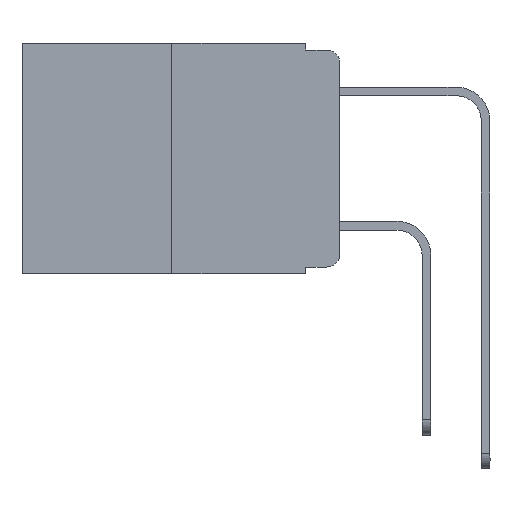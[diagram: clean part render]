
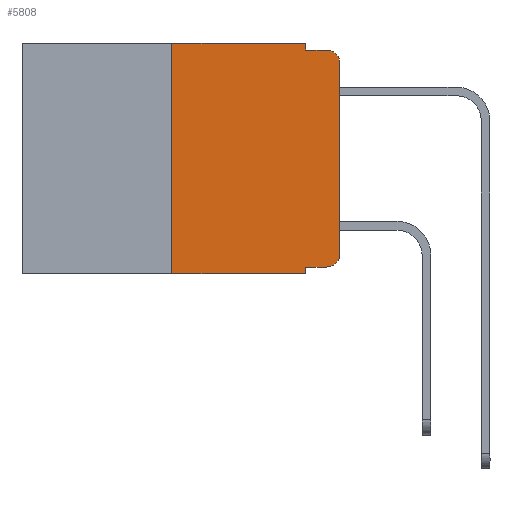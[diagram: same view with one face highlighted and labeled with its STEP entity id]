
A CAD part, left-side view. The second image highlights one B-rep face of the part: STEP entity #5808.
In plain terms, the highlighted planar face has unit normal (-1, 0, 0).
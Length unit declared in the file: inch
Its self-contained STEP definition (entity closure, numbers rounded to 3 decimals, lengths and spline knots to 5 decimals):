
#131 = CARTESIAN_POINT ( 'NONE',  ( 0., 0.02, -0.333 ) ) ;
#281 = CARTESIAN_POINT ( 'NONE',  ( 0., 0.473, 0. ) ) ;
#1119 = DIRECTION ( 'NONE',  ( 0., -1., 0. ) ) ;
#1161 = LINE ( 'NONE', #17422, #10593 ) ;
#2213 = EDGE_CURVE ( 'NONE', #14482, #23473, #11950, .T. ) ;
#2402 = EDGE_CURVE ( 'NONE', #11995, #22808, #20182, .T. ) ;
#2594 = VECTOR ( 'NONE', #10227, 39.37008 ) ;
#2926 = DIRECTION ( 'NONE',  ( 0., 0., -1. ) ) ;
#3239 = EDGE_CURVE ( 'NONE', #14482, #4214, #15384, .T. ) ;
#3507 = VECTOR ( 'NONE', #1119, 39.37008 ) ;
#3679 = CARTESIAN_POINT ( 'NONE',  ( 0., 0.051, -0.333 ) ) ;
#3742 = CIRCLE ( 'NONE', #18759, 0.02 ) ;
#4099 = VERTEX_POINT ( 'NONE', #24246 ) ;
#4214 = VERTEX_POINT ( 'NONE', #25661 ) ;
#5206 = DIRECTION ( 'NONE',  ( 0., 0., -1. ) ) ;
#5703 = LINE ( 'NONE', #21969, #22738 ) ;
#5708 = ORIENTED_EDGE ( 'NONE', *, *, #2402, .T. ) ;
#5808 = ADVANCED_FACE ( 'NONE', ( #22714 ), #18697, .F. ) ;
#6368 = ORIENTED_EDGE ( 'NONE', *, *, #11559, .F. ) ;
#6681 = VECTOR ( 'NONE', #22497, 39.37008 ) ;
#6683 = EDGE_CURVE ( 'NONE', #16133, #4099, #24520, .T. ) ;
#7158 = CARTESIAN_POINT ( 'NONE',  ( 0., 0.051, -0.01 ) ) ;
#7384 = ORIENTED_EDGE ( 'NONE', *, *, #6683, .F. ) ;
#7598 = DIRECTION ( 'NONE',  ( 0., 0., -1. ) ) ;
#8269 = VECTOR ( 'NONE', #2926, 39.37008 ) ;
#8389 = VERTEX_POINT ( 'NONE', #9646 ) ;
#8846 = ORIENTED_EDGE ( 'NONE', *, *, #21223, .F. ) ;
#9257 = CARTESIAN_POINT ( 'NONE',  ( 0., 0.02, -0.03 ) ) ;
#9646 = CARTESIAN_POINT ( 'NONE',  ( 0., 0., -0.313 ) ) ;
#9952 = CARTESIAN_POINT ( 'NONE',  ( 0., 0.051, -0.333 ) ) ;
#10069 = EDGE_LOOP ( 'NONE', ( #24864, #5708, #21512, #6368, #7384, #8846, #12903, #10584, #22811, #16232 ) ) ;
#10111 = DIRECTION ( 'NONE',  ( 0., 0., -1. ) ) ;
#10227 = DIRECTION ( 'NONE',  ( 0., -1., 0. ) ) ;
#10337 = EDGE_CURVE ( 'NONE', #22990, #22808, #19526, .T. ) ;
#10584 = ORIENTED_EDGE ( 'NONE', *, *, #3239, .F. ) ;
#10593 = VECTOR ( 'NONE', #23998, 39.37008 ) ;
#11559 = EDGE_CURVE ( 'NONE', #4099, #22990, #5703, .T. ) ;
#11950 = LINE ( 'NONE', #9952, #2594 ) ;
#11995 = VERTEX_POINT ( 'NONE', #26079 ) ;
#12903 = ORIENTED_EDGE ( 'NONE', *, *, #26313, .T. ) ;
#13415 = DIRECTION ( 'NONE',  ( 0., 0., 1. ) ) ;
#13844 = VECTOR ( 'NONE', #13415, 39.37008 ) ;
#14438 = LINE ( 'NONE', #19959, #25424 ) ;
#14482 = VERTEX_POINT ( 'NONE', #3679 ) ;
#15384 = LINE ( 'NONE', #23603, #8269 ) ;
#15413 = LINE ( 'NONE', #23634, #13844 ) ;
#15506 = DIRECTION ( 'NONE',  ( 0., 0., -1. ) ) ;
#15543 = DIRECTION ( 'NONE',  ( -1., 0., 0. ) ) ;
#16031 = AXIS2_PLACEMENT_3D ( 'NONE', #281, #24481, #10111 ) ;
#16133 = VERTEX_POINT ( 'NONE', #19725 ) ;
#16232 = ORIENTED_EDGE ( 'NONE', *, *, #25167, .T. ) ;
#16446 = CARTESIAN_POINT ( 'NONE',  ( 0., 0.473, 0. ) ) ;
#17422 = CARTESIAN_POINT ( 'NONE',  ( 0., 0.473, -0.343 ) ) ;
#17816 = CARTESIAN_POINT ( 'NONE',  ( 0., 0.02, -0.313 ) ) ;
#18697 = PLANE ( 'NONE',  #16031 ) ;
#18759 = AXIS2_PLACEMENT_3D ( 'NONE', #17816, #26019, #7598 ) ;
#19340 = EDGE_CURVE ( 'NONE', #8389, #11995, #15413, .T. ) ;
#19526 = LINE ( 'NONE', #7158, #3507 ) ;
#19725 = CARTESIAN_POINT ( 'NONE',  ( 0., 0.25, 0. ) ) ;
#19959 = CARTESIAN_POINT ( 'NONE',  ( 0., 0.25, 0. ) ) ;
#20088 = DIRECTION ( 'NONE',  ( 0., 0., 1. ) ) ;
#20182 = CIRCLE ( 'NONE', #26208, 0.02 ) ;
#20976 = CARTESIAN_POINT ( 'NONE',  ( 0., 0.051, -0.01 ) ) ;
#21223 = EDGE_CURVE ( 'NONE', #23189, #16133, #14438, .T. ) ;
#21512 = ORIENTED_EDGE ( 'NONE', *, *, #10337, .F. ) ;
#21969 = CARTESIAN_POINT ( 'NONE',  ( 0., 0.051, 0. ) ) ;
#22497 = DIRECTION ( 'NONE',  ( 0., -1., 0. ) ) ;
#22714 = FACE_OUTER_BOUND ( 'NONE', #10069, .T. ) ;
#22738 = VECTOR ( 'NONE', #15506, 39.37008 ) ;
#22808 = VERTEX_POINT ( 'NONE', #25442 ) ;
#22811 = ORIENTED_EDGE ( 'NONE', *, *, #2213, .T. ) ;
#22990 = VERTEX_POINT ( 'NONE', #20976 ) ;
#23189 = VERTEX_POINT ( 'NONE', #23521 ) ;
#23473 = VERTEX_POINT ( 'NONE', #131 ) ;
#23521 = CARTESIAN_POINT ( 'NONE',  ( 0., 0.25, -0.343 ) ) ;
#23603 = CARTESIAN_POINT ( 'NONE',  ( 0., 0.051, 0. ) ) ;
#23634 = CARTESIAN_POINT ( 'NONE',  ( 0., 0., 0. ) ) ;
#23998 = DIRECTION ( 'NONE',  ( 0., -1., 0. ) ) ;
#24246 = CARTESIAN_POINT ( 'NONE',  ( 0., 0.051, 0. ) ) ;
#24481 = DIRECTION ( 'NONE',  ( 1., 0., 0. ) ) ;
#24520 = LINE ( 'NONE', #16446, #6681 ) ;
#24864 = ORIENTED_EDGE ( 'NONE', *, *, #19340, .T. ) ;
#25167 = EDGE_CURVE ( 'NONE', #23473, #8389, #3742, .T. ) ;
#25424 = VECTOR ( 'NONE', #20088, 39.37008 ) ;
#25442 = CARTESIAN_POINT ( 'NONE',  ( 0., 0.02, -0.01 ) ) ;
#25661 = CARTESIAN_POINT ( 'NONE',  ( 0., 0.051, -0.343 ) ) ;
#26019 = DIRECTION ( 'NONE',  ( -1., 0., 0. ) ) ;
#26079 = CARTESIAN_POINT ( 'NONE',  ( 0., 0., -0.03 ) ) ;
#26208 = AXIS2_PLACEMENT_3D ( 'NONE', #9257, #15543, #5206 ) ;
#26313 = EDGE_CURVE ( 'NONE', #23189, #4214, #1161, .T. ) ;
